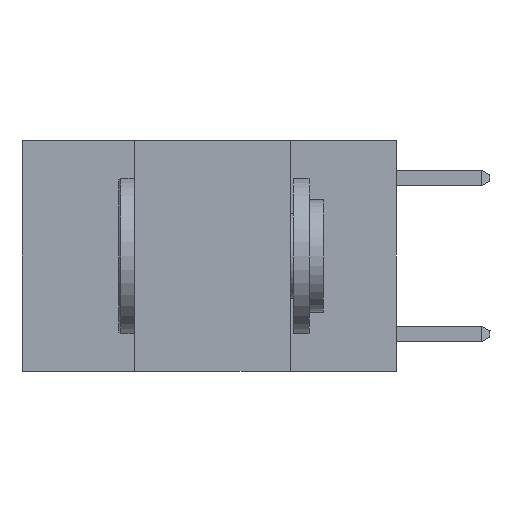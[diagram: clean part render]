
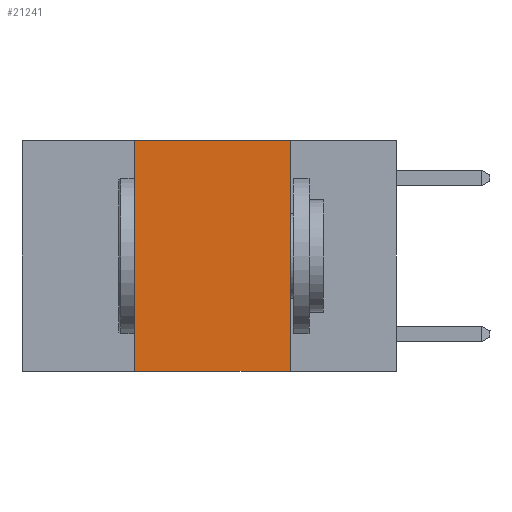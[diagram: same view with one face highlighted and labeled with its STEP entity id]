
A CAD part, left-side view. The second image highlights one B-rep face of the part: STEP entity #21241.
In plain terms, the highlighted planar face has unit normal (-1, 0, 0).
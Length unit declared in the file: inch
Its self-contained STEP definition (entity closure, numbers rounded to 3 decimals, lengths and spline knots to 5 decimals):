
#425 = AXIS2_PLACEMENT_3D ( 'NONE', #8038, #25266, #10562 ) ;
#1758 = LINE ( 'NONE', #25741, #22355 ) ;
#2842 = CARTESIAN_POINT ( 'NONE',  ( 0., 0.42, -0.37 ) ) ;
#3436 = CARTESIAN_POINT ( 'NONE',  ( 0., 0.6, -0.37 ) ) ;
#3940 = VECTOR ( 'NONE', #13395, 39.37008 ) ;
#5969 = DIRECTION ( 'NONE',  ( 0., -1., 0. ) ) ;
#7244 = VERTEX_POINT ( 'NONE', #24833 ) ;
#8038 = CARTESIAN_POINT ( 'NONE',  ( 0., 0.6, 0. ) ) ;
#8765 = VECTOR ( 'NONE', #5969, 39.37008 ) ;
#10562 = DIRECTION ( 'NONE',  ( 0., 0., -1. ) ) ;
#10744 = EDGE_CURVE ( 'NONE', #17689, #29291, #22009, .T. ) ;
#10909 = CARTESIAN_POINT ( 'NONE',  ( 0., 0.17, 0. ) ) ;
#11041 = CARTESIAN_POINT ( 'NONE',  ( 0., 0.42, 0. ) ) ;
#13395 = DIRECTION ( 'NONE',  ( 0., 0., -1. ) ) ;
#13743 = CARTESIAN_POINT ( 'NONE',  ( 0., 0.42, 0. ) ) ;
#14661 = EDGE_CURVE ( 'NONE', #17689, #7244, #15375, .T. ) ;
#14695 = EDGE_LOOP ( 'NONE', ( #20304, #20469, #20607, #20838 ) ) ;
#15375 = LINE ( 'NONE', #3436, #8765 ) ;
#16243 = VERTEX_POINT ( 'NONE', #19779 ) ;
#17689 = VERTEX_POINT ( 'NONE', #2842 ) ;
#18492 = DIRECTION ( 'NONE',  ( 0., -1., 0. ) ) ;
#19779 = CARTESIAN_POINT ( 'NONE',  ( 0., 0.17, 0. ) ) ;
#20304 = ORIENTED_EDGE ( 'NONE', *, *, #20754, .F. ) ;
#20361 = PLANE ( 'NONE',  #425 ) ;
#20469 = ORIENTED_EDGE ( 'NONE', *, *, #29298, .F. ) ;
#20607 = ORIENTED_EDGE ( 'NONE', *, *, #10744, .F. ) ;
#20754 = EDGE_CURVE ( 'NONE', #16243, #7244, #22898, .T. ) ;
#20838 = ORIENTED_EDGE ( 'NONE', *, *, #14661, .T. ) ;
#20952 = FACE_OUTER_BOUND ( 'NONE', #14695, .T. ) ;
#21241 = ADVANCED_FACE ( 'NONE', ( #20952 ), #20361, .F. ) ;
#21258 = VECTOR ( 'NONE', #26045, 39.37008 ) ;
#22009 = LINE ( 'NONE', #13743, #21258 ) ;
#22355 = VECTOR ( 'NONE', #18492, 39.37008 ) ;
#22898 = LINE ( 'NONE', #10909, #3940 ) ;
#24833 = CARTESIAN_POINT ( 'NONE',  ( 0., 0.17, -0.37 ) ) ;
#25266 = DIRECTION ( 'NONE',  ( 1., 0., 0. ) ) ;
#25741 = CARTESIAN_POINT ( 'NONE',  ( 0., 0.6, 0. ) ) ;
#26045 = DIRECTION ( 'NONE',  ( 0., 0., 1. ) ) ;
#29291 = VERTEX_POINT ( 'NONE', #11041 ) ;
#29298 = EDGE_CURVE ( 'NONE', #29291, #16243, #1758, .T. ) ;
